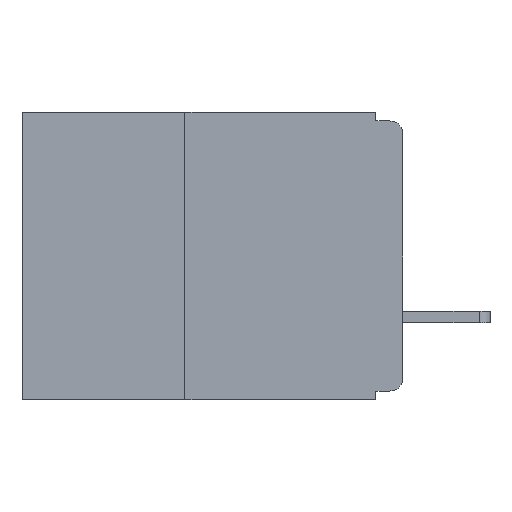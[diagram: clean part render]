
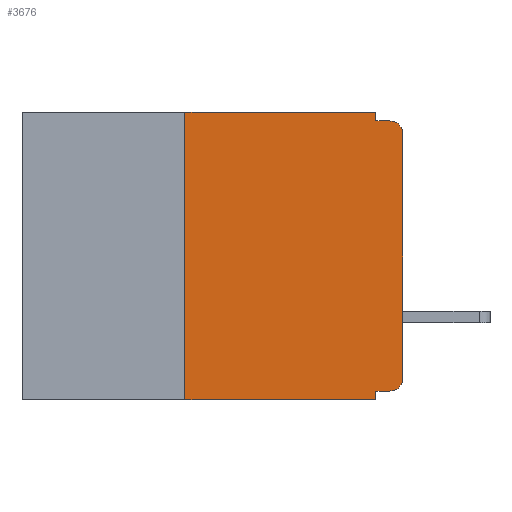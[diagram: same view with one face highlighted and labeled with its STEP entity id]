
A CAD part, left-side view. The second image highlights one B-rep face of the part: STEP entity #3676.
In plain terms, the highlighted planar face has unit normal (-1, 0, 0).
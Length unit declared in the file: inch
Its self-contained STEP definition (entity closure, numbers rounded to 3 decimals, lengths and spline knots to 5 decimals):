
#3 = ORIENTED_EDGE ( 'NONE', *, *, #15728, .F. ) ;
#194 = ORIENTED_EDGE ( 'NONE', *, *, #3898, .F. ) ;
#197 = ORIENTED_EDGE ( 'NONE', *, *, #14621, .F. ) ;
#271 = ORIENTED_EDGE ( 'NONE', *, *, #7879, .T. ) ;
#293 = ORIENTED_EDGE ( 'NONE', *, *, #7453, .F. ) ;
#298 = VECTOR ( 'NONE', #10857, 39.37008 ) ;
#350 = ORIENTED_EDGE ( 'NONE', *, *, #4496, .F. ) ;
#430 = VERTEX_POINT ( 'NONE', #11535 ) ;
#628 = ORIENTED_EDGE ( 'NONE', *, *, #6095, .T. ) ;
#867 = CARTESIAN_POINT ( 'NONE',  ( 0., 0.437, 0. ) ) ;
#1035 = CARTESIAN_POINT ( 'NONE',  ( 0., 0.437, -0.33 ) ) ;
#1140 = DIRECTION ( 'NONE',  ( 0., -1., 0. ) ) ;
#1375 = DIRECTION ( 'NONE',  ( 0., -1., 0. ) ) ;
#1513 = AXIS2_PLACEMENT_3D ( 'NONE', #11863, #11587, #11469 ) ;
#2234 = CARTESIAN_POINT ( 'NONE',  ( 0., 0., -0.025 ) ) ;
#2469 = VECTOR ( 'NONE', #1375, 39.37008 ) ;
#2521 = LINE ( 'NONE', #1035, #2469 ) ;
#2580 = EDGE_LOOP ( 'NONE', ( #15885, #15859, #15799, #3, #194, #197, #271, #293, #350, #628 ) ) ;
#2616 = DIRECTION ( 'NONE',  ( 0., 0., -1. ) ) ;
#2986 = DIRECTION ( 'NONE',  ( -1., 0., 0. ) ) ;
#3011 = CIRCLE ( 'NONE', #9423, 0.015 ) ;
#3122 = CARTESIAN_POINT ( 'NONE',  ( 0., 0.015, -0.025 ) ) ;
#3385 = VECTOR ( 'NONE', #13732, 39.37008 ) ;
#3388 = VECTOR ( 'NONE', #12246, 39.37008 ) ;
#3455 = CARTESIAN_POINT ( 'NONE',  ( 0., 0.015, -0.32 ) ) ;
#3590 = LINE ( 'NONE', #13685, #3385 ) ;
#3676 = ADVANCED_FACE ( 'NONE', ( #8249 ), #11673, .F. ) ;
#3716 = LINE ( 'NONE', #12936, #3388 ) ;
#3894 = CARTESIAN_POINT ( 'NONE',  ( 0., 0.031, -0.32 ) ) ;
#3898 = EDGE_CURVE ( 'NONE', #11835, #13052, #15193, .T. ) ;
#4489 = AXIS2_PLACEMENT_3D ( 'NONE', #6759, #6587, #6584 ) ;
#4496 = EDGE_CURVE ( 'NONE', #6904, #8395, #5469, .T. ) ;
#4935 = VECTOR ( 'NONE', #7780, 39.37008 ) ;
#4943 = LINE ( 'NONE', #6083, #4935 ) ;
#5078 = VERTEX_POINT ( 'NONE', #9019 ) ;
#5469 = LINE ( 'NONE', #10945, #298 ) ;
#6083 = CARTESIAN_POINT ( 'NONE',  ( 0., 0., -0.01 ) ) ;
#6095 = EDGE_CURVE ( 'NONE', #6904, #5078, #7928, .T. ) ;
#6526 = CARTESIAN_POINT ( 'NONE',  ( 0., 0.031, -0.01 ) ) ;
#6584 = DIRECTION ( 'NONE',  ( 0., 0., -1. ) ) ;
#6587 = DIRECTION ( 'NONE',  ( -1., 0., 0. ) ) ;
#6759 = CARTESIAN_POINT ( 'NONE',  ( 0., 0.015, -0.305 ) ) ;
#6904 = VERTEX_POINT ( 'NONE', #3455 ) ;
#7453 = EDGE_CURVE ( 'NONE', #8395, #10821, #3716, .T. ) ;
#7780 = DIRECTION ( 'NONE',  ( 0., -1., 0. ) ) ;
#7822 = VERTEX_POINT ( 'NONE', #2234 ) ;
#7879 = EDGE_CURVE ( 'NONE', #9236, #10821, #2521, .T. ) ;
#7928 = CIRCLE ( 'NONE', #4489, 0.015 ) ;
#8249 = FACE_OUTER_BOUND ( 'NONE', #2580, .T. ) ;
#8395 = VERTEX_POINT ( 'NONE', #3894 ) ;
#8676 = CARTESIAN_POINT ( 'NONE',  ( 0., 0.25, -0.33 ) ) ;
#9019 = CARTESIAN_POINT ( 'NONE',  ( 0., 0., -0.305 ) ) ;
#9236 = VERTEX_POINT ( 'NONE', #8676 ) ;
#9423 = AXIS2_PLACEMENT_3D ( 'NONE', #3122, #2986, #2616 ) ;
#9793 = EDGE_CURVE ( 'NONE', #5078, #7822, #11170, .T. ) ;
#10821 = VERTEX_POINT ( 'NONE', #13235 ) ;
#10857 = DIRECTION ( 'NONE',  ( 0., 1., 0. ) ) ;
#10945 = CARTESIAN_POINT ( 'NONE',  ( 0., 0., -0.32 ) ) ;
#11129 = VECTOR ( 'NONE', #12313, 39.37008 ) ;
#11170 = LINE ( 'NONE', #12409, #11129 ) ;
#11469 = DIRECTION ( 'NONE',  ( 0., 0., -1. ) ) ;
#11535 = CARTESIAN_POINT ( 'NONE',  ( 0., 0.015, -0.01 ) ) ;
#11587 = DIRECTION ( 'NONE',  ( 1., 0., 0. ) ) ;
#11673 = PLANE ( 'NONE',  #1513 ) ;
#11711 = EDGE_CURVE ( 'NONE', #7822, #430, #3011, .T. ) ;
#11835 = VERTEX_POINT ( 'NONE', #16478 ) ;
#11863 = CARTESIAN_POINT ( 'NONE',  ( 0., 0.437, 0. ) ) ;
#12246 = DIRECTION ( 'NONE',  ( 0., 0., -1. ) ) ;
#12255 = VERTEX_POINT ( 'NONE', #6526 ) ;
#12313 = DIRECTION ( 'NONE',  ( 0., 0., 1. ) ) ;
#12409 = CARTESIAN_POINT ( 'NONE',  ( 0., 0., 0. ) ) ;
#12936 = CARTESIAN_POINT ( 'NONE',  ( 0., 0.031, -0.33 ) ) ;
#13052 = VERTEX_POINT ( 'NONE', #14214 ) ;
#13235 = CARTESIAN_POINT ( 'NONE',  ( 0., 0.031, -0.33 ) ) ;
#13685 = CARTESIAN_POINT ( 'NONE',  ( 0., 0.25, -0.33 ) ) ;
#13732 = DIRECTION ( 'NONE',  ( 0., 0., 1. ) ) ;
#14214 = CARTESIAN_POINT ( 'NONE',  ( 0., 0.031, 0. ) ) ;
#14330 = EDGE_CURVE ( 'NONE', #12255, #430, #4943, .T. ) ;
#14621 = EDGE_CURVE ( 'NONE', #9236, #11835, #3590, .T. ) ;
#14961 = VECTOR ( 'NONE', #15777, 39.37008 ) ;
#15035 = VECTOR ( 'NONE', #1140, 39.37008 ) ;
#15110 = LINE ( 'NONE', #16077, #14961 ) ;
#15193 = LINE ( 'NONE', #867, #15035 ) ;
#15728 = EDGE_CURVE ( 'NONE', #13052, #12255, #15110, .T. ) ;
#15777 = DIRECTION ( 'NONE',  ( 0., 0., -1. ) ) ;
#15799 = ORIENTED_EDGE ( 'NONE', *, *, #14330, .F. ) ;
#15859 = ORIENTED_EDGE ( 'NONE', *, *, #11711, .T. ) ;
#15885 = ORIENTED_EDGE ( 'NONE', *, *, #9793, .T. ) ;
#16077 = CARTESIAN_POINT ( 'NONE',  ( 0., 0.031, 0. ) ) ;
#16478 = CARTESIAN_POINT ( 'NONE',  ( 0., 0.25, 0. ) ) ;
